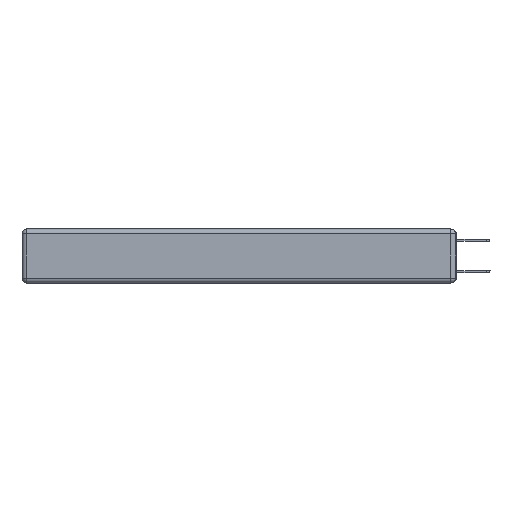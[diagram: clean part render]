
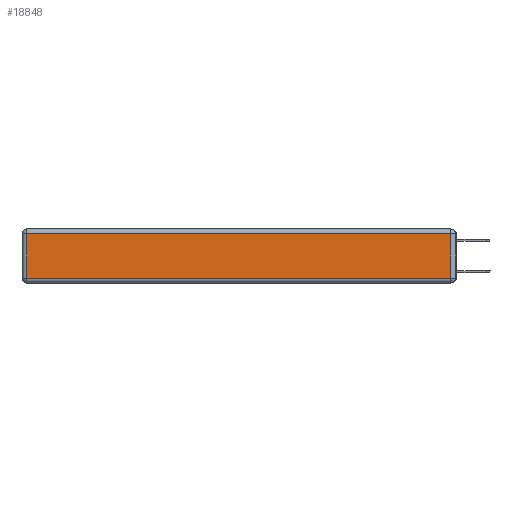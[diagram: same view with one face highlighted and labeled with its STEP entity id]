
A CAD part, left-side view. The second image highlights one B-rep face of the part: STEP entity #18848.
In plain terms, the highlighted planar face has unit normal (-1, 0, 0).
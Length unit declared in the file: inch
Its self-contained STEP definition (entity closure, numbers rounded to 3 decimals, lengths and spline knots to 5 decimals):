
#1522 = DIRECTION ( 'NONE',  ( -1., 0., 0. ) ) ;
#1946 = EDGE_CURVE ( 'NONE', #7863, #9583, #19909, .T. ) ;
#2083 = VECTOR ( 'NONE', #10463, 39.37008 ) ;
#3853 = DIRECTION ( 'NONE',  ( 0., 1., 0. ) ) ;
#3863 = LINE ( 'NONE', #13051, #13373 ) ;
#4733 = CARTESIAN_POINT ( 'NONE',  ( 0., 2.72, -0.343 ) ) ;
#5789 = CARTESIAN_POINT ( 'NONE',  ( 0., 0.03, -0.343 ) ) ;
#7372 = DIRECTION ( 'NONE',  ( 0., 0., 1. ) ) ;
#7462 = ORIENTED_EDGE ( 'NONE', *, *, #14703, .T. ) ;
#7863 = VERTEX_POINT ( 'NONE', #10289 ) ;
#8829 = FACE_OUTER_BOUND ( 'NONE', #15245, .T. ) ;
#9221 = CARTESIAN_POINT ( 'NONE',  ( 0., 0.03, -0.03 ) ) ;
#9583 = VERTEX_POINT ( 'NONE', #9221 ) ;
#9715 = DIRECTION ( 'NONE',  ( 0., 0., -1. ) ) ;
#10289 = CARTESIAN_POINT ( 'NONE',  ( 0., 0.03, -0.313 ) ) ;
#10463 = DIRECTION ( 'NONE',  ( 0., -1., 0. ) ) ;
#10621 = CARTESIAN_POINT ( 'NONE',  ( 0., 2.72, -0.313 ) ) ;
#11002 = ORIENTED_EDGE ( 'NONE', *, *, #11310, .T. ) ;
#11310 = EDGE_CURVE ( 'NONE', #9583, #19490, #3863, .T. ) ;
#12492 = CARTESIAN_POINT ( 'NONE',  ( 0., 0., -0.343 ) ) ;
#13051 = CARTESIAN_POINT ( 'NONE',  ( 0., 2.75, -0.03 ) ) ;
#13373 = VECTOR ( 'NONE', #3853, 39.37008 ) ;
#13994 = ORIENTED_EDGE ( 'NONE', *, *, #16306, .T. ) ;
#14703 = EDGE_CURVE ( 'NONE', #19490, #15837, #17120, .T. ) ;
#14938 = VECTOR ( 'NONE', #9715, 39.37008 ) ;
#15245 = EDGE_LOOP ( 'NONE', ( #13994, #16238, #11002, #7462 ) ) ;
#15772 = VECTOR ( 'NONE', #7372, 39.37008 ) ;
#15837 = VERTEX_POINT ( 'NONE', #10621 ) ;
#16238 = ORIENTED_EDGE ( 'NONE', *, *, #1946, .T. ) ;
#16306 = EDGE_CURVE ( 'NONE', #15837, #7863, #19652, .T. ) ;
#16572 = CARTESIAN_POINT ( 'NONE',  ( 0., 0., -0.313 ) ) ;
#16820 = AXIS2_PLACEMENT_3D ( 'NONE', #12492, #1522, #20177 ) ;
#17120 = LINE ( 'NONE', #4733, #14938 ) ;
#17179 = PLANE ( 'NONE',  #16820 ) ;
#18848 = ADVANCED_FACE ( 'NONE', ( #8829 ), #17179, .T. ) ;
#19490 = VERTEX_POINT ( 'NONE', #19959 ) ;
#19652 = LINE ( 'NONE', #16572, #2083 ) ;
#19909 = LINE ( 'NONE', #5789, #15772 ) ;
#19959 = CARTESIAN_POINT ( 'NONE',  ( 0., 2.72, -0.03 ) ) ;
#20177 = DIRECTION ( 'NONE',  ( 0., 0., 1. ) ) ;
